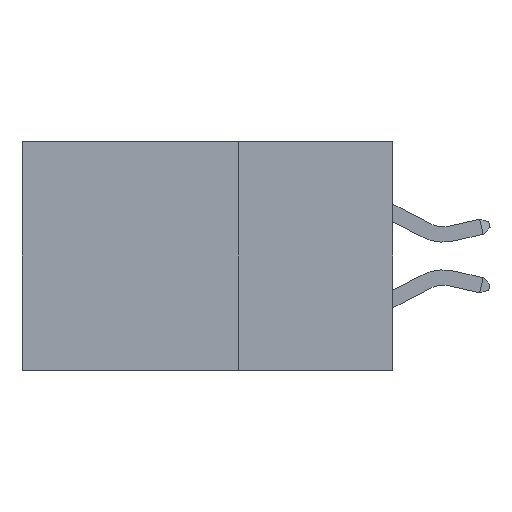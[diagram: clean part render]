
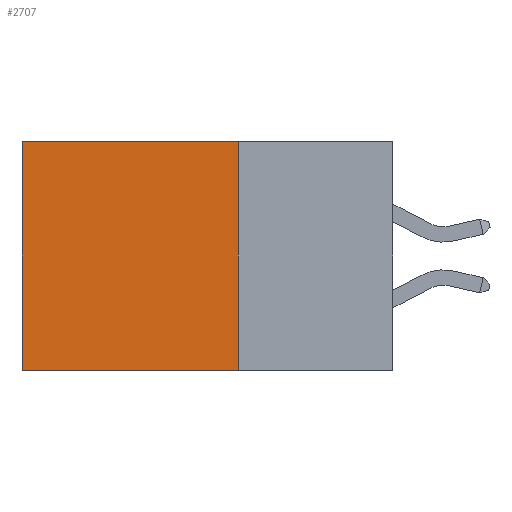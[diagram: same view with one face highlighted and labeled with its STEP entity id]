
A CAD part, left-side view. The second image highlights one B-rep face of the part: STEP entity #2707.
In plain terms, the highlighted planar face has unit normal (-1, 0, 0).
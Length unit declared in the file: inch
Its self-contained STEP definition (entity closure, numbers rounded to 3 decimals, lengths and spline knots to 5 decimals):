
#246 = EDGE_CURVE ( 'NONE', #531, #5574, #3118, .T. ) ;
#386 = DIRECTION ( 'NONE',  ( 0., 0., -1. ) ) ;
#484 = DIRECTION ( 'NONE',  ( 0., 0., -1. ) ) ;
#531 = VERTEX_POINT ( 'NONE', #3426 ) ;
#541 = CARTESIAN_POINT ( 'NONE',  ( 0.2875, 0.6, 0. ) ) ;
#1205 = CARTESIAN_POINT ( 'NONE',  ( 0.2875, 0.25, -0.37 ) ) ;
#1253 = DIRECTION ( 'NONE',  ( 1., 0., 0. ) ) ;
#1293 = DIRECTION ( 'NONE',  ( 0., 1., 0. ) ) ;
#1354 = ORIENTED_EDGE ( 'NONE', *, *, #10074, .T. ) ;
#1491 = CARTESIAN_POINT ( 'NONE',  ( 0.2875, 0.6, 0. ) ) ;
#1679 = VECTOR ( 'NONE', #1293, 39.37008 ) ;
#2131 = PLANE ( 'NONE',  #5423 ) ;
#2488 = CARTESIAN_POINT ( 'NONE',  ( 0.2875, 0.25, 0. ) ) ;
#2707 = ADVANCED_FACE ( 'NONE', ( #5670 ), #2131, .F. ) ;
#3118 = LINE ( 'NONE', #1205, #10190 ) ;
#3426 = CARTESIAN_POINT ( 'NONE',  ( 0.2875, 0.25, -0.37 ) ) ;
#4019 = CARTESIAN_POINT ( 'NONE',  ( 0.2875, 0.25, 0. ) ) ;
#4370 = VECTOR ( 'NONE', #9491, 39.37008 ) ;
#4870 = DIRECTION ( 'NONE',  ( 0., 1., 0. ) ) ;
#5377 = VECTOR ( 'NONE', #484, 39.37008 ) ;
#5423 = AXIS2_PLACEMENT_3D ( 'NONE', #9244, #1253, #386 ) ;
#5574 = VERTEX_POINT ( 'NONE', #11136 ) ;
#5670 = FACE_OUTER_BOUND ( 'NONE', #5987, .T. ) ;
#5987 = EDGE_LOOP ( 'NONE', ( #7967, #10565, #8896, #1354 ) ) ;
#6078 = LINE ( 'NONE', #2488, #4370 ) ;
#7915 = EDGE_CURVE ( 'NONE', #8338, #531, #6078, .T. ) ;
#7967 = ORIENTED_EDGE ( 'NONE', *, *, #8706, .T. ) ;
#7998 = CARTESIAN_POINT ( 'NONE',  ( 0.2875, 0.25, 0. ) ) ;
#8338 = VERTEX_POINT ( 'NONE', #7998 ) ;
#8469 = LINE ( 'NONE', #541, #5377 ) ;
#8706 = EDGE_CURVE ( 'NONE', #9767, #5574, #8469, .T. ) ;
#8896 = ORIENTED_EDGE ( 'NONE', *, *, #7915, .F. ) ;
#9244 = CARTESIAN_POINT ( 'NONE',  ( 0.2875, 0.25, 0. ) ) ;
#9283 = LINE ( 'NONE', #4019, #1679 ) ;
#9491 = DIRECTION ( 'NONE',  ( 0., 0., -1. ) ) ;
#9767 = VERTEX_POINT ( 'NONE', #1491 ) ;
#10074 = EDGE_CURVE ( 'NONE', #8338, #9767, #9283, .T. ) ;
#10190 = VECTOR ( 'NONE', #4870, 39.37008 ) ;
#10565 = ORIENTED_EDGE ( 'NONE', *, *, #246, .F. ) ;
#11136 = CARTESIAN_POINT ( 'NONE',  ( 0.2875, 0.6, -0.37 ) ) ;
